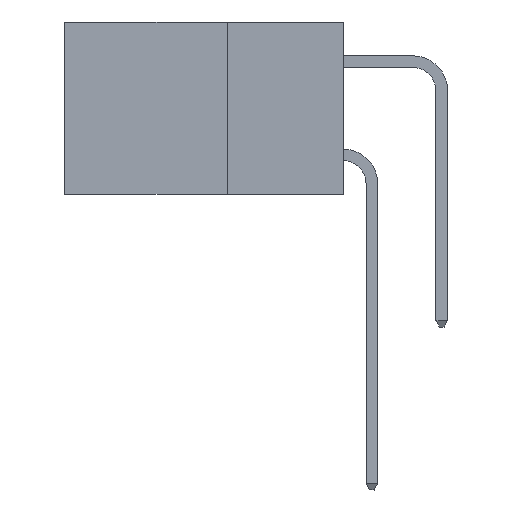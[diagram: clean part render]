
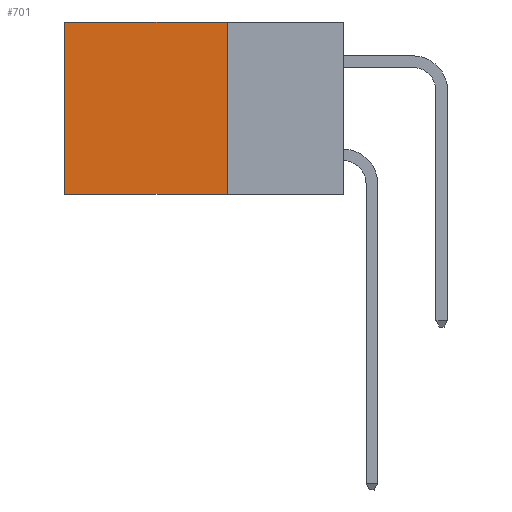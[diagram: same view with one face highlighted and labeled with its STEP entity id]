
A CAD part, left-side view. The second image highlights one B-rep face of the part: STEP entity #701.
In plain terms, the highlighted planar face has unit normal (-1, 0, 0).
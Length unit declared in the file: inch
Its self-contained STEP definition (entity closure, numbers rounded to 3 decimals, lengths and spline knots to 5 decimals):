
#458 = EDGE_CURVE ( 'NONE', #28126, #657, #681, .T. ) ;
#502 = DIRECTION ( 'NONE',  ( 0., 0., -1. ) ) ;
#564 = VECTOR ( 'NONE', #19652, 39.37008 ) ;
#657 = VERTEX_POINT ( 'NONE', #25788 ) ;
#681 = LINE ( 'NONE', #27421, #5814 ) ;
#701 = ADVANCED_FACE ( 'NONE', ( #10079 ), #26082, .F. ) ;
#959 = DIRECTION ( 'NONE',  ( 0., 0., -1. ) ) ;
#2548 = LINE ( 'NONE', #11380, #18458 ) ;
#5600 = EDGE_CURVE ( 'NONE', #28126, #16998, #2548, .T. ) ;
#5814 = VECTOR ( 'NONE', #23154, 39.37008 ) ;
#6138 = ORIENTED_EDGE ( 'NONE', *, *, #8832, .T. ) ;
#6299 = AXIS2_PLACEMENT_3D ( 'NONE', #12710, #21672, #959 ) ;
#8832 = EDGE_CURVE ( 'NONE', #657, #28899, #15116, .T. ) ;
#10079 = FACE_OUTER_BOUND ( 'NONE', #13297, .T. ) ;
#10877 = ORIENTED_EDGE ( 'NONE', *, *, #13130, .F. ) ;
#11380 = CARTESIAN_POINT ( 'NONE',  ( 0.2615, 0.25, -0.37 ) ) ;
#11975 = VECTOR ( 'NONE', #25975, 39.37008 ) ;
#12710 = CARTESIAN_POINT ( 'NONE',  ( 0.2615, 0.25, -0.37 ) ) ;
#13130 = EDGE_CURVE ( 'NONE', #16998, #28899, #19234, .T. ) ;
#13297 = EDGE_LOOP ( 'NONE', ( #6138, #10877, #13766, #20615 ) ) ;
#13766 = ORIENTED_EDGE ( 'NONE', *, *, #5600, .F. ) ;
#15116 = LINE ( 'NONE', #17009, #564 ) ;
#15451 = CARTESIAN_POINT ( 'NONE',  ( 0.2615, 0.6, -0.37 ) ) ;
#16998 = VERTEX_POINT ( 'NONE', #27768 ) ;
#17009 = CARTESIAN_POINT ( 'NONE',  ( 0.2615, 0.6, -0.37 ) ) ;
#17014 = CARTESIAN_POINT ( 'NONE',  ( 0.2615, 0.25, -0.37 ) ) ;
#18458 = VECTOR ( 'NONE', #502, 39.37008 ) ;
#19234 = LINE ( 'NONE', #17014, #11975 ) ;
#19652 = DIRECTION ( 'NONE',  ( 0., 0., -1. ) ) ;
#20615 = ORIENTED_EDGE ( 'NONE', *, *, #458, .T. ) ;
#21672 = DIRECTION ( 'NONE',  ( 1., 0., 0. ) ) ;
#23154 = DIRECTION ( 'NONE',  ( 0., 1., 0. ) ) ;
#25788 = CARTESIAN_POINT ( 'NONE',  ( 0.2615, 0.6, 0. ) ) ;
#25975 = DIRECTION ( 'NONE',  ( 0., 1., 0. ) ) ;
#26082 = PLANE ( 'NONE',  #6299 ) ;
#26677 = CARTESIAN_POINT ( 'NONE',  ( 0.2615, 0.25, 0. ) ) ;
#27421 = CARTESIAN_POINT ( 'NONE',  ( 0.2615, 0.25, 0. ) ) ;
#27768 = CARTESIAN_POINT ( 'NONE',  ( 0.2615, 0.25, -0.37 ) ) ;
#28126 = VERTEX_POINT ( 'NONE', #26677 ) ;
#28899 = VERTEX_POINT ( 'NONE', #15451 ) ;
